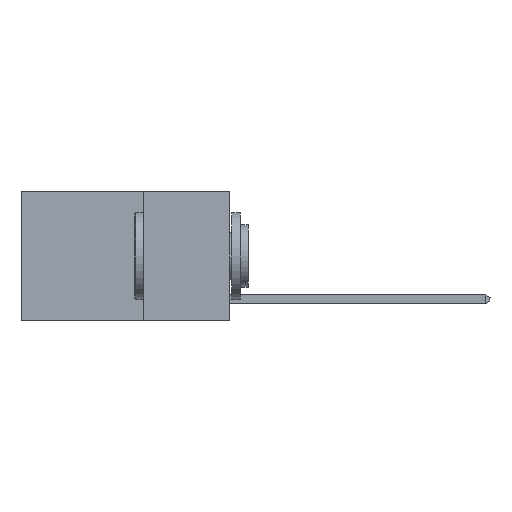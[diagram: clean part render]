
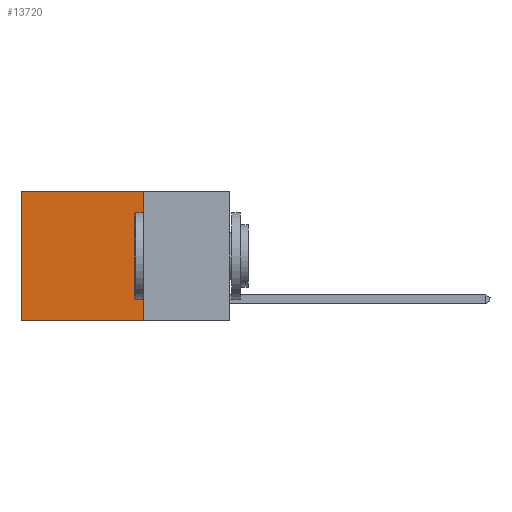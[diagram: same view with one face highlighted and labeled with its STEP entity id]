
A CAD part, left-side view. The second image highlights one B-rep face of the part: STEP entity #13720.
In plain terms, the highlighted planar face has unit normal (-1, 0, 0).
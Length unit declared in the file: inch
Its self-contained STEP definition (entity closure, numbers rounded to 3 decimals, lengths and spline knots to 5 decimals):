
#670 = AXIS2_PLACEMENT_3D ( 'NONE', #14862, #7904, #903 ) ;
#903 = DIRECTION ( 'NONE',  ( 0., 0., -1. ) ) ;
#1199 = VECTOR ( 'NONE', #12758, 39.37008 ) ;
#1713 = CARTESIAN_POINT ( 'NONE',  ( 0.2625, 0.25, 0. ) ) ;
#1797 = DIRECTION ( 'NONE',  ( 0., 0., -1. ) ) ;
#2098 = ORIENTED_EDGE ( 'NONE', *, *, #5887, .F. ) ;
#2333 = ORIENTED_EDGE ( 'NONE', *, *, #3672, .T. ) ;
#2419 = LINE ( 'NONE', #7732, #11026 ) ;
#2449 = CARTESIAN_POINT ( 'NONE',  ( 0.2625, 0.6, -0.37 ) ) ;
#2766 = VERTEX_POINT ( 'NONE', #2449 ) ;
#2820 = VECTOR ( 'NONE', #14736, 39.37008 ) ;
#2856 = VERTEX_POINT ( 'NONE', #11017 ) ;
#3672 = EDGE_CURVE ( 'NONE', #10734, #2766, #10881, .T. ) ;
#3859 = EDGE_LOOP ( 'NONE', ( #2333, #7182, #2098, #11008 ) ) ;
#4741 = CARTESIAN_POINT ( 'NONE',  ( 0.2625, 0.25, 0. ) ) ;
#5428 = CARTESIAN_POINT ( 'NONE',  ( 0.2625, 0.6, 0. ) ) ;
#5887 = EDGE_CURVE ( 'NONE', #13940, #2856, #6983, .T. ) ;
#6688 = PLANE ( 'NONE',  #670 ) ;
#6983 = LINE ( 'NONE', #1713, #10079 ) ;
#7182 = ORIENTED_EDGE ( 'NONE', *, *, #9452, .F. ) ;
#7398 = FACE_OUTER_BOUND ( 'NONE', #3859, .T. ) ;
#7732 = CARTESIAN_POINT ( 'NONE',  ( 0.2625, 0.25, 0. ) ) ;
#7785 = DIRECTION ( 'NONE',  ( 0., 1., 0. ) ) ;
#7904 = DIRECTION ( 'NONE',  ( 1., 0., 0. ) ) ;
#9452 = EDGE_CURVE ( 'NONE', #2856, #2766, #12152, .T. ) ;
#10079 = VECTOR ( 'NONE', #1797, 39.37008 ) ;
#10734 = VERTEX_POINT ( 'NONE', #5428 ) ;
#10881 = LINE ( 'NONE', #12902, #1199 ) ;
#11008 = ORIENTED_EDGE ( 'NONE', *, *, #14319, .T. ) ;
#11017 = CARTESIAN_POINT ( 'NONE',  ( 0.2625, 0.25, -0.37 ) ) ;
#11026 = VECTOR ( 'NONE', #7785, 39.37008 ) ;
#12152 = LINE ( 'NONE', #13537, #2820 ) ;
#12758 = DIRECTION ( 'NONE',  ( 0., 0., -1. ) ) ;
#12902 = CARTESIAN_POINT ( 'NONE',  ( 0.2625, 0.6, 0. ) ) ;
#13537 = CARTESIAN_POINT ( 'NONE',  ( 0.2625, 0.25, -0.37 ) ) ;
#13720 = ADVANCED_FACE ( 'NONE', ( #7398 ), #6688, .F. ) ;
#13940 = VERTEX_POINT ( 'NONE', #4741 ) ;
#14319 = EDGE_CURVE ( 'NONE', #13940, #10734, #2419, .T. ) ;
#14736 = DIRECTION ( 'NONE',  ( 0., 1., 0. ) ) ;
#14862 = CARTESIAN_POINT ( 'NONE',  ( 0.2625, 0.25, 0. ) ) ;
